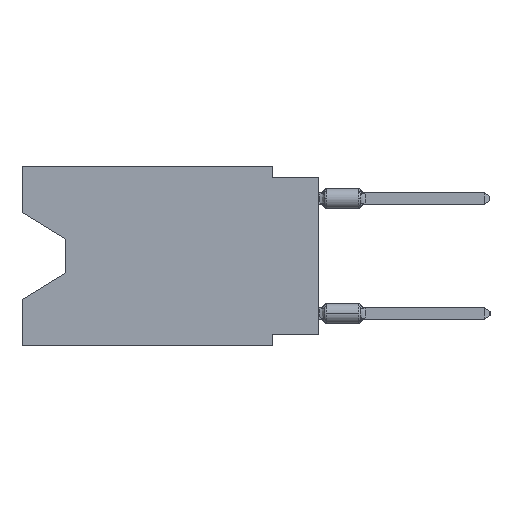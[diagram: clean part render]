
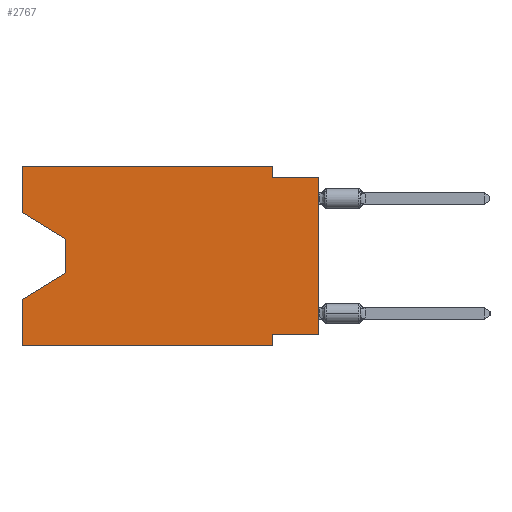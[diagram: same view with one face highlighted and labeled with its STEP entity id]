
A CAD part, left-side view. The second image highlights one B-rep face of the part: STEP entity #2767.
In plain terms, the highlighted planar face has unit normal (-1, 0, 0).
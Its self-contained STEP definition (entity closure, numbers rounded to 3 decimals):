
#230 = CARTESIAN_POINT ( 'NONE',  ( 0., 2.54, 0. ) ) ;
#811 = LINE ( 'NONE', #11332, #14564 ) ;
#1065 = VECTOR ( 'NONE', #19649, 1000. ) ;
#1097 = VERTEX_POINT ( 'NONE', #10898 ) ;
#1739 = CARTESIAN_POINT ( 'NONE',  ( 0., 2.54, -9.271 ) ) ;
#2134 = DIRECTION ( 'NONE',  ( 1., 0., 0. ) ) ;
#2767 = ADVANCED_FACE ( 'NONE', ( #14316 ), #16908, .F. ) ;
#2966 = DIRECTION ( 'NONE',  ( 0., 0., -1. ) ) ;
#3278 = VERTEX_POINT ( 'NONE', #18732 ) ;
#3546 = EDGE_CURVE ( 'NONE', #27208, #28602, #20599, .T. ) ;
#4276 = VERTEX_POINT ( 'NONE', #1739 ) ;
#4933 = VECTOR ( 'NONE', #30402, 1000. ) ;
#5664 = CARTESIAN_POINT ( 'NONE',  ( 0., 16.383, -2.546 ) ) ;
#7401 = EDGE_CURVE ( 'NONE', #19537, #27208, #14040, .T. ) ;
#7417 = EDGE_CURVE ( 'NONE', #19537, #9946, #23825, .T. ) ;
#8701 = CARTESIAN_POINT ( 'NONE',  ( 0., 16.383, 0. ) ) ;
#9001 = CARTESIAN_POINT ( 'NONE',  ( 0., 16.383, -9.906 ) ) ;
#9149 = LINE ( 'NONE', #16722, #1065 ) ;
#9600 = CARTESIAN_POINT ( 'NONE',  ( 0., 0., -0.635 ) ) ;
#9837 = CARTESIAN_POINT ( 'NONE',  ( 0., 16.383, -9.906 ) ) ;
#9946 = VERTEX_POINT ( 'NONE', #32174 ) ;
#10019 = CARTESIAN_POINT ( 'NONE',  ( 0., 0., -9.271 ) ) ;
#10097 = CARTESIAN_POINT ( 'NONE',  ( 0., 16.383, 0. ) ) ;
#10112 = ORIENTED_EDGE ( 'NONE', *, *, #25826, .F. ) ;
#10773 = CARTESIAN_POINT ( 'NONE',  ( 0., 16.383, -2.546 ) ) ;
#10877 = VERTEX_POINT ( 'NONE', #27981 ) ;
#10898 = CARTESIAN_POINT ( 'NONE',  ( 0., 2.54, -0.635 ) ) ;
#11218 = EDGE_CURVE ( 'NONE', #10877, #16392, #25697, .T. ) ;
#11332 = CARTESIAN_POINT ( 'NONE',  ( 0., 2.54, -9.906 ) ) ;
#12184 = CARTESIAN_POINT ( 'NONE',  ( 0., 16.383, 0. ) ) ;
#12376 = VECTOR ( 'NONE', #25942, 1000. ) ;
#12485 = CARTESIAN_POINT ( 'NONE',  ( 0., 13.97, -5.893 ) ) ;
#13678 = CARTESIAN_POINT ( 'NONE',  ( 0., 16.383, -7.36 ) ) ;
#13760 = ORIENTED_EDGE ( 'NONE', *, *, #15117, .T. ) ;
#14040 = LINE ( 'NONE', #8701, #28896 ) ;
#14316 = FACE_OUTER_BOUND ( 'NONE', #28083, .T. ) ;
#14564 = VECTOR ( 'NONE', #21818, 1000. ) ;
#15117 = EDGE_CURVE ( 'NONE', #9946, #10877, #9149, .T. ) ;
#15154 = VECTOR ( 'NONE', #20607, 1000. ) ;
#15369 = ORIENTED_EDGE ( 'NONE', *, *, #3546, .F. ) ;
#15467 = LINE ( 'NONE', #23385, #12376 ) ;
#15626 = EDGE_CURVE ( 'NONE', #19757, #32995, #20612, .T. ) ;
#15742 = DIRECTION ( 'NONE',  ( 0., 0., -1. ) ) ;
#16392 = VERTEX_POINT ( 'NONE', #13678 ) ;
#16526 = ORIENTED_EDGE ( 'NONE', *, *, #31477, .F. ) ;
#16722 = CARTESIAN_POINT ( 'NONE',  ( 0., 13.97, -4.013 ) ) ;
#16908 = PLANE ( 'NONE',  #27748 ) ;
#17286 = ORIENTED_EDGE ( 'NONE', *, *, #7417, .T. ) ;
#17691 = CARTESIAN_POINT ( 'NONE',  ( 0., 0., 0. ) ) ;
#17857 = DIRECTION ( 'NONE',  ( 0., -1., 0. ) ) ;
#18007 = EDGE_CURVE ( 'NONE', #4276, #3278, #811, .T. ) ;
#18694 = EDGE_CURVE ( 'NONE', #1097, #32995, #15467, .T. ) ;
#18696 = VECTOR ( 'NONE', #20332, 1000. ) ;
#18732 = CARTESIAN_POINT ( 'NONE',  ( 0., 2.54, -9.906 ) ) ;
#19196 = DIRECTION ( 'NONE',  ( 0., 0., 1. ) ) ;
#19537 = VERTEX_POINT ( 'NONE', #5664 ) ;
#19649 = DIRECTION ( 'NONE',  ( 0., 0., -1. ) ) ;
#19757 = VERTEX_POINT ( 'NONE', #19796 ) ;
#19796 = CARTESIAN_POINT ( 'NONE',  ( 0., 0., -9.271 ) ) ;
#20332 = DIRECTION ( 'NONE',  ( 0., -1., 0. ) ) ;
#20599 = LINE ( 'NONE', #12184, #26685 ) ;
#20607 = DIRECTION ( 'NONE',  ( 0., 0., 1. ) ) ;
#20612 = LINE ( 'NONE', #17691, #4933 ) ;
#21268 = DIRECTION ( 'NONE',  ( 0., -0.855, -0.519 ) ) ;
#21818 = DIRECTION ( 'NONE',  ( 0., 0., -1. ) ) ;
#22889 = CARTESIAN_POINT ( 'NONE',  ( 0., 16.383, 0. ) ) ;
#22959 = DIRECTION ( 'NONE',  ( 0., 0.855, -0.519 ) ) ;
#23141 = EDGE_CURVE ( 'NONE', #28602, #1097, #26549, .T. ) ;
#23179 = LINE ( 'NONE', #10097, #15154 ) ;
#23385 = CARTESIAN_POINT ( 'NONE',  ( 0., 0., -0.635 ) ) ;
#23825 = LINE ( 'NONE', #10773, #30534 ) ;
#24693 = VECTOR ( 'NONE', #28451, 1000. ) ;
#24992 = VECTOR ( 'NONE', #2966, 1000. ) ;
#25697 = LINE ( 'NONE', #12485, #30588 ) ;
#25826 = EDGE_CURVE ( 'NONE', #19757, #4276, #31188, .T. ) ;
#25942 = DIRECTION ( 'NONE',  ( 0., -1., 0. ) ) ;
#26109 = ORIENTED_EDGE ( 'NONE', *, *, #23141, .F. ) ;
#26281 = ORIENTED_EDGE ( 'NONE', *, *, #26872, .T. ) ;
#26549 = LINE ( 'NONE', #230, #24992 ) ;
#26685 = VECTOR ( 'NONE', #17857, 1000. ) ;
#26777 = ORIENTED_EDGE ( 'NONE', *, *, #18694, .F. ) ;
#26872 = EDGE_CURVE ( 'NONE', #30788, #3278, #30653, .T. ) ;
#27208 = VERTEX_POINT ( 'NONE', #22889 ) ;
#27382 = CARTESIAN_POINT ( 'NONE',  ( 0., 16.383, 0. ) ) ;
#27748 = AXIS2_PLACEMENT_3D ( 'NONE', #27382, #2134, #15742 ) ;
#27981 = CARTESIAN_POINT ( 'NONE',  ( 0., 13.97, -5.893 ) ) ;
#28083 = EDGE_LOOP ( 'NONE', ( #17286, #13760, #32486, #16526, #26281, #33410, #10112, #31191, #26777, #26109, #15369, #33923 ) ) ;
#28451 = DIRECTION ( 'NONE',  ( 0., 1., 0. ) ) ;
#28602 = VERTEX_POINT ( 'NONE', #32313 ) ;
#28896 = VECTOR ( 'NONE', #19196, 1000. ) ;
#30402 = DIRECTION ( 'NONE',  ( 0., 0., 1. ) ) ;
#30534 = VECTOR ( 'NONE', #21268, 1000. ) ;
#30588 = VECTOR ( 'NONE', #22959, 1000. ) ;
#30653 = LINE ( 'NONE', #9837, #18696 ) ;
#30788 = VERTEX_POINT ( 'NONE', #9001 ) ;
#31188 = LINE ( 'NONE', #10019, #24693 ) ;
#31191 = ORIENTED_EDGE ( 'NONE', *, *, #15626, .T. ) ;
#31477 = EDGE_CURVE ( 'NONE', #30788, #16392, #23179, .T. ) ;
#32174 = CARTESIAN_POINT ( 'NONE',  ( 0., 13.97, -4.013 ) ) ;
#32313 = CARTESIAN_POINT ( 'NONE',  ( 0., 2.54, 0. ) ) ;
#32486 = ORIENTED_EDGE ( 'NONE', *, *, #11218, .T. ) ;
#32995 = VERTEX_POINT ( 'NONE', #9600 ) ;
#33410 = ORIENTED_EDGE ( 'NONE', *, *, #18007, .F. ) ;
#33923 = ORIENTED_EDGE ( 'NONE', *, *, #7401, .F. ) ;
